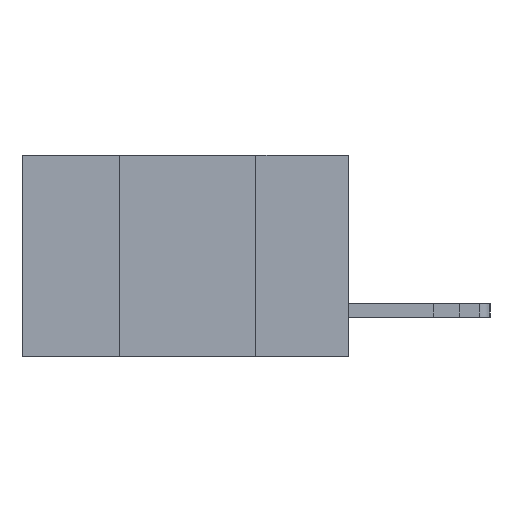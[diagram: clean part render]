
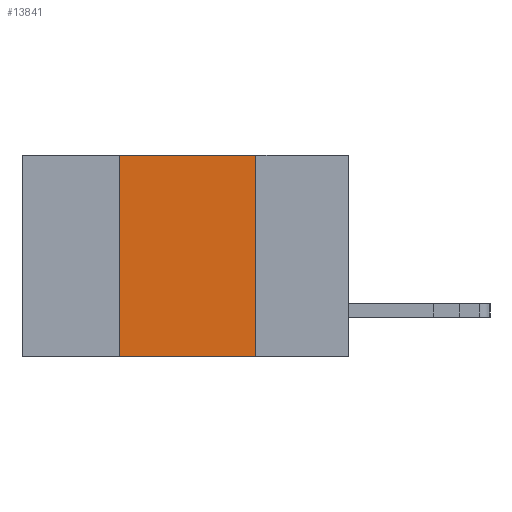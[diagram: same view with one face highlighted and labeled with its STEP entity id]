
A CAD part, left-side view. The second image highlights one B-rep face of the part: STEP entity #13841.
In plain terms, the highlighted planar face has unit normal (-1, 0, 0).
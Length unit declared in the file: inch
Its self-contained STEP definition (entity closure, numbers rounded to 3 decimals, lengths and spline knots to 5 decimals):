
#369 = LINE ( 'NONE', #1775, #6634 ) ;
#626 = CARTESIAN_POINT ( 'NONE',  ( 0., 0.17, -0.37 ) ) ;
#1775 = CARTESIAN_POINT ( 'NONE',  ( 0., 0.6, 0. ) ) ;
#1875 = ORIENTED_EDGE ( 'NONE', *, *, #13002, .T. ) ;
#2264 = ORIENTED_EDGE ( 'NONE', *, *, #6173, .F. ) ;
#2685 = EDGE_CURVE ( 'NONE', #14047, #6003, #369, .T. ) ;
#2999 = VERTEX_POINT ( 'NONE', #12236 ) ;
#3044 = PLANE ( 'NONE',  #4498 ) ;
#4336 = DIRECTION ( 'NONE',  ( 0., 0., -1. ) ) ;
#4498 = AXIS2_PLACEMENT_3D ( 'NONE', #15260, #11703, #4336 ) ;
#5209 = CARTESIAN_POINT ( 'NONE',  ( 0., 0.6, -0.37 ) ) ;
#5565 = CARTESIAN_POINT ( 'NONE',  ( 0., 0.42, 0. ) ) ;
#5582 = VERTEX_POINT ( 'NONE', #626 ) ;
#5944 = CARTESIAN_POINT ( 'NONE',  ( 0., 0.42, 0. ) ) ;
#6003 = VERTEX_POINT ( 'NONE', #8967 ) ;
#6173 = EDGE_CURVE ( 'NONE', #2999, #14047, #6645, .T. ) ;
#6358 = FACE_OUTER_BOUND ( 'NONE', #13400, .T. ) ;
#6634 = VECTOR ( 'NONE', #9280, 39.37008 ) ;
#6645 = LINE ( 'NONE', #5565, #15906 ) ;
#6690 = LINE ( 'NONE', #13859, #12596 ) ;
#8967 = CARTESIAN_POINT ( 'NONE',  ( 0., 0.17, 0. ) ) ;
#9039 = DIRECTION ( 'NONE',  ( 0., 0., -1. ) ) ;
#9280 = DIRECTION ( 'NONE',  ( 0., -1., 0. ) ) ;
#10299 = EDGE_CURVE ( 'NONE', #6003, #5582, #6690, .T. ) ;
#11182 = ORIENTED_EDGE ( 'NONE', *, *, #10299, .F. ) ;
#11703 = DIRECTION ( 'NONE',  ( 1., 0., 0. ) ) ;
#12236 = CARTESIAN_POINT ( 'NONE',  ( 0., 0.42, -0.37 ) ) ;
#12466 = LINE ( 'NONE', #5209, #15286 ) ;
#12596 = VECTOR ( 'NONE', #9039, 39.37008 ) ;
#12911 = DIRECTION ( 'NONE',  ( 0., 0., 1. ) ) ;
#13002 = EDGE_CURVE ( 'NONE', #2999, #5582, #12466, .T. ) ;
#13266 = ORIENTED_EDGE ( 'NONE', *, *, #2685, .F. ) ;
#13400 = EDGE_LOOP ( 'NONE', ( #11182, #13266, #2264, #1875 ) ) ;
#13841 = ADVANCED_FACE ( 'NONE', ( #6358 ), #3044, .F. ) ;
#13859 = CARTESIAN_POINT ( 'NONE',  ( 0., 0.17, 0. ) ) ;
#14047 = VERTEX_POINT ( 'NONE', #5944 ) ;
#14912 = DIRECTION ( 'NONE',  ( 0., -1., 0. ) ) ;
#15260 = CARTESIAN_POINT ( 'NONE',  ( 0., 0.6, 0. ) ) ;
#15286 = VECTOR ( 'NONE', #14912, 39.37008 ) ;
#15906 = VECTOR ( 'NONE', #12911, 39.37008 ) ;
